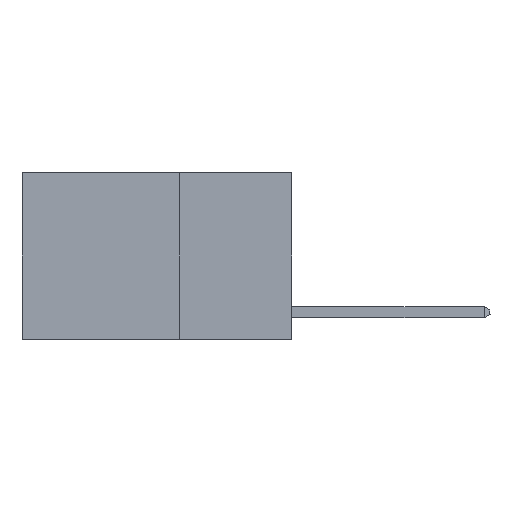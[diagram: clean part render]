
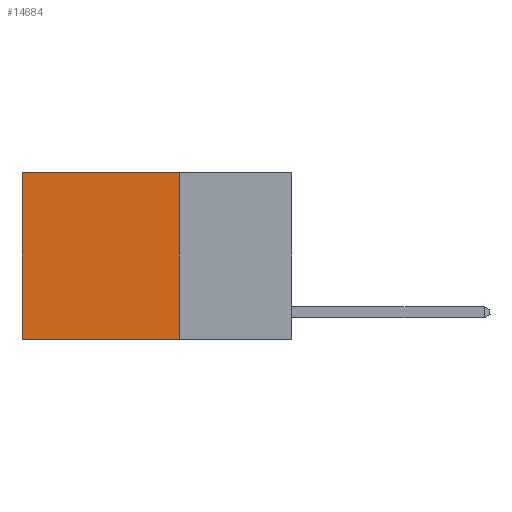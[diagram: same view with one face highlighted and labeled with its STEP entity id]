
A CAD part, left-side view. The second image highlights one B-rep face of the part: STEP entity #14684.
In plain terms, the highlighted planar face has unit normal (-1, 0, 0).
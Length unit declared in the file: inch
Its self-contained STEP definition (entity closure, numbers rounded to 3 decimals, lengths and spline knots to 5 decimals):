
#345 = VECTOR ( 'NONE', #2612, 39.37008 ) ;
#1424 = EDGE_CURVE ( 'NONE', #5178, #21825, #18993, .T. ) ;
#2602 = LINE ( 'NONE', #15805, #21324 ) ;
#2612 = DIRECTION ( 'NONE',  ( 0., 1., 0. ) ) ;
#2622 = DIRECTION ( 'NONE',  ( 0., 0., -1. ) ) ;
#3039 = EDGE_CURVE ( 'NONE', #10373, #8276, #20885, .T. ) ;
#3525 = EDGE_LOOP ( 'NONE', ( #5707, #4775, #23236, #8156 ) ) ;
#3583 = CARTESIAN_POINT ( 'NONE',  ( 0.2625, 0.6, -0.37 ) ) ;
#4430 = DIRECTION ( 'NONE',  ( 0., 0., -1. ) ) ;
#4513 = LINE ( 'NONE', #18995, #19028 ) ;
#4775 = ORIENTED_EDGE ( 'NONE', *, *, #3039, .F. ) ;
#5178 = VERTEX_POINT ( 'NONE', #16384 ) ;
#5707 = ORIENTED_EDGE ( 'NONE', *, *, #21459, .T. ) ;
#6189 = DIRECTION ( 'NONE',  ( 0., 1., 0. ) ) ;
#6203 = EDGE_CURVE ( 'NONE', #5178, #10373, #4513, .T. ) ;
#8156 = ORIENTED_EDGE ( 'NONE', *, *, #1424, .T. ) ;
#8276 = VERTEX_POINT ( 'NONE', #3583 ) ;
#10185 = CARTESIAN_POINT ( 'NONE',  ( 0.2625, 0.6, 0. ) ) ;
#10373 = VERTEX_POINT ( 'NONE', #23288 ) ;
#11546 = CARTESIAN_POINT ( 'NONE',  ( 0.2625, 0.25, -0.37 ) ) ;
#12143 = DIRECTION ( 'NONE',  ( 0., 0., -1. ) ) ;
#13108 = AXIS2_PLACEMENT_3D ( 'NONE', #13583, #13252, #4430 ) ;
#13252 = DIRECTION ( 'NONE',  ( 1., 0., 0. ) ) ;
#13583 = CARTESIAN_POINT ( 'NONE',  ( 0.2625, 0.25, 0. ) ) ;
#13903 = CARTESIAN_POINT ( 'NONE',  ( 0.2625, 0.25, 0. ) ) ;
#14501 = VECTOR ( 'NONE', #6189, 39.37008 ) ;
#14684 = ADVANCED_FACE ( 'NONE', ( #15254 ), #22833, .F. ) ;
#15254 = FACE_OUTER_BOUND ( 'NONE', #3525, .T. ) ;
#15805 = CARTESIAN_POINT ( 'NONE',  ( 0.2625, 0.6, 0. ) ) ;
#16384 = CARTESIAN_POINT ( 'NONE',  ( 0.2625, 0.25, 0. ) ) ;
#18993 = LINE ( 'NONE', #13903, #345 ) ;
#18995 = CARTESIAN_POINT ( 'NONE',  ( 0.2625, 0.25, 0. ) ) ;
#19028 = VECTOR ( 'NONE', #2622, 39.37008 ) ;
#20885 = LINE ( 'NONE', #11546, #14501 ) ;
#21324 = VECTOR ( 'NONE', #12143, 39.37008 ) ;
#21459 = EDGE_CURVE ( 'NONE', #21825, #8276, #2602, .T. ) ;
#21825 = VERTEX_POINT ( 'NONE', #10185 ) ;
#22833 = PLANE ( 'NONE',  #13108 ) ;
#23236 = ORIENTED_EDGE ( 'NONE', *, *, #6203, .F. ) ;
#23288 = CARTESIAN_POINT ( 'NONE',  ( 0.2625, 0.25, -0.37 ) ) ;
